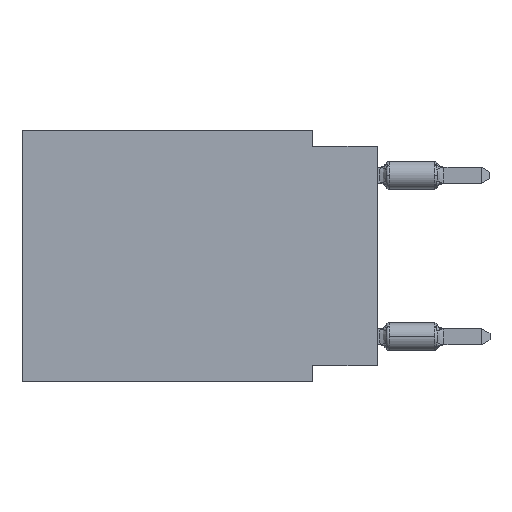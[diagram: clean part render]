
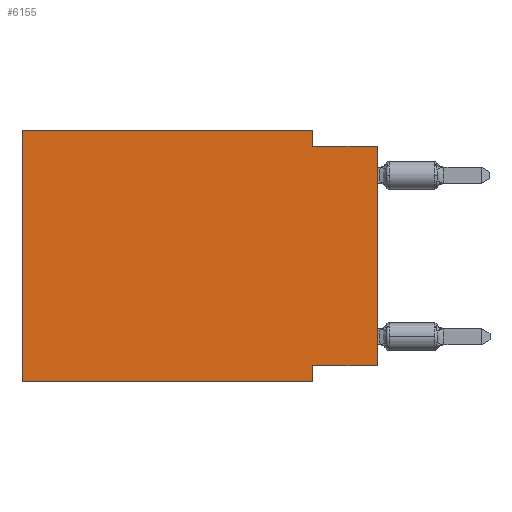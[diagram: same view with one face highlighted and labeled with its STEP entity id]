
A CAD part, left-side view. The second image highlights one B-rep face of the part: STEP entity #6155.
In plain terms, the highlighted planar face has unit normal (-1, 0, 0).
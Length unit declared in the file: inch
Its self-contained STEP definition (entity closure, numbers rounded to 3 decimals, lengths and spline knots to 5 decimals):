
#174 = CARTESIAN_POINT ( 'NONE',  ( 0., 0.1, -0.365 ) ) ;
#357 = VECTOR ( 'NONE', #4681, 39.37008 ) ;
#507 = VECTOR ( 'NONE', #9048, 39.37008 ) ;
#508 = ORIENTED_EDGE ( 'NONE', *, *, #8563, .F. ) ;
#656 = CARTESIAN_POINT ( 'NONE',  ( 0., 0.1, 0. ) ) ;
#1331 = CARTESIAN_POINT ( 'NONE',  ( 0., 0., -0.025 ) ) ;
#1517 = CARTESIAN_POINT ( 'NONE',  ( 0., 0.55, 0. ) ) ;
#1786 = VECTOR ( 'NONE', #5687, 39.37008 ) ;
#1942 = DIRECTION ( 'NONE',  ( 0., 0., 1. ) ) ;
#2149 = VERTEX_POINT ( 'NONE', #11740 ) ;
#2542 = VERTEX_POINT ( 'NONE', #8471 ) ;
#2840 = CARTESIAN_POINT ( 'NONE',  ( 0., 0.55, 0. ) ) ;
#2858 = VERTEX_POINT ( 'NONE', #1331 ) ;
#3270 = EDGE_CURVE ( 'NONE', #2149, #12677, #6531, .T. ) ;
#3497 = AXIS2_PLACEMENT_3D ( 'NONE', #2840, #7424, #4218 ) ;
#3628 = DIRECTION ( 'NONE',  ( 0., 0., 1. ) ) ;
#3714 = VECTOR ( 'NONE', #5478, 39.37008 ) ;
#3947 = CARTESIAN_POINT ( 'NONE',  ( 0., 0.55, -0.39 ) ) ;
#3995 = LINE ( 'NONE', #12900, #8737 ) ;
#4218 = DIRECTION ( 'NONE',  ( 0., 0., -1. ) ) ;
#4255 = ORIENTED_EDGE ( 'NONE', *, *, #5894, .F. ) ;
#4501 = ORIENTED_EDGE ( 'NONE', *, *, #6526, .F. ) ;
#4629 = LINE ( 'NONE', #8622, #1786 ) ;
#4681 = DIRECTION ( 'NONE',  ( 0., 0., -1. ) ) ;
#4911 = EDGE_LOOP ( 'NONE', ( #10481, #4255, #8327, #508, #11575, #12512, #9215, #4501 ) ) ;
#4946 = EDGE_CURVE ( 'NONE', #2149, #9110, #11797, .T. ) ;
#4990 = CARTESIAN_POINT ( 'NONE',  ( 0., 0., -0.365 ) ) ;
#5347 = EDGE_CURVE ( 'NONE', #10309, #2858, #10927, .T. ) ;
#5478 = DIRECTION ( 'NONE',  ( 0., -1., 0. ) ) ;
#5543 = VECTOR ( 'NONE', #3628, 39.37008 ) ;
#5545 = LINE ( 'NONE', #656, #357 ) ;
#5687 = DIRECTION ( 'NONE',  ( 0., 0., -1. ) ) ;
#5894 = EDGE_CURVE ( 'NONE', #2542, #2858, #6083, .T. ) ;
#5944 = EDGE_CURVE ( 'NONE', #8721, #9110, #4629, .T. ) ;
#6083 = LINE ( 'NONE', #12082, #12035 ) ;
#6155 = ADVANCED_FACE ( 'NONE', ( #7835 ), #11817, .F. ) ;
#6526 = EDGE_CURVE ( 'NONE', #10309, #8721, #3995, .T. ) ;
#6531 = LINE ( 'NONE', #1517, #5543 ) ;
#7131 = DIRECTION ( 'NONE',  ( 0., -1., 0. ) ) ;
#7424 = DIRECTION ( 'NONE',  ( 1., 0., 0. ) ) ;
#7835 = FACE_OUTER_BOUND ( 'NONE', #4911, .T. ) ;
#8327 = ORIENTED_EDGE ( 'NONE', *, *, #8617, .F. ) ;
#8471 = CARTESIAN_POINT ( 'NONE',  ( 0., 0.1, -0.025 ) ) ;
#8563 = EDGE_CURVE ( 'NONE', #12677, #10653, #12606, .T. ) ;
#8617 = EDGE_CURVE ( 'NONE', #10653, #2542, #5545, .T. ) ;
#8622 = CARTESIAN_POINT ( 'NONE',  ( 0., 0.1, -0.39 ) ) ;
#8721 = VERTEX_POINT ( 'NONE', #174 ) ;
#8737 = VECTOR ( 'NONE', #11912, 39.37008 ) ;
#8846 = CARTESIAN_POINT ( 'NONE',  ( 0., 0., 0. ) ) ;
#9048 = DIRECTION ( 'NONE',  ( 0., -1., 0. ) ) ;
#9110 = VERTEX_POINT ( 'NONE', #12956 ) ;
#9215 = ORIENTED_EDGE ( 'NONE', *, *, #5944, .F. ) ;
#9371 = CARTESIAN_POINT ( 'NONE',  ( 0., 0.1, 0. ) ) ;
#9461 = CARTESIAN_POINT ( 'NONE',  ( 0., 0.55, 0. ) ) ;
#9727 = VECTOR ( 'NONE', #1942, 39.37008 ) ;
#10309 = VERTEX_POINT ( 'NONE', #4990 ) ;
#10481 = ORIENTED_EDGE ( 'NONE', *, *, #5347, .T. ) ;
#10653 = VERTEX_POINT ( 'NONE', #9371 ) ;
#10927 = LINE ( 'NONE', #8846, #9727 ) ;
#11575 = ORIENTED_EDGE ( 'NONE', *, *, #3270, .F. ) ;
#11666 = CARTESIAN_POINT ( 'NONE',  ( 0., 0.55, 0. ) ) ;
#11740 = CARTESIAN_POINT ( 'NONE',  ( 0., 0.55, -0.39 ) ) ;
#11797 = LINE ( 'NONE', #3947, #507 ) ;
#11817 = PLANE ( 'NONE',  #3497 ) ;
#11912 = DIRECTION ( 'NONE',  ( 0., 1., 0. ) ) ;
#12035 = VECTOR ( 'NONE', #7131, 39.37008 ) ;
#12082 = CARTESIAN_POINT ( 'NONE',  ( 0., 0., -0.025 ) ) ;
#12512 = ORIENTED_EDGE ( 'NONE', *, *, #4946, .T. ) ;
#12606 = LINE ( 'NONE', #9461, #3714 ) ;
#12677 = VERTEX_POINT ( 'NONE', #11666 ) ;
#12900 = CARTESIAN_POINT ( 'NONE',  ( 0., 0., -0.365 ) ) ;
#12956 = CARTESIAN_POINT ( 'NONE',  ( 0., 0.1, -0.39 ) ) ;
